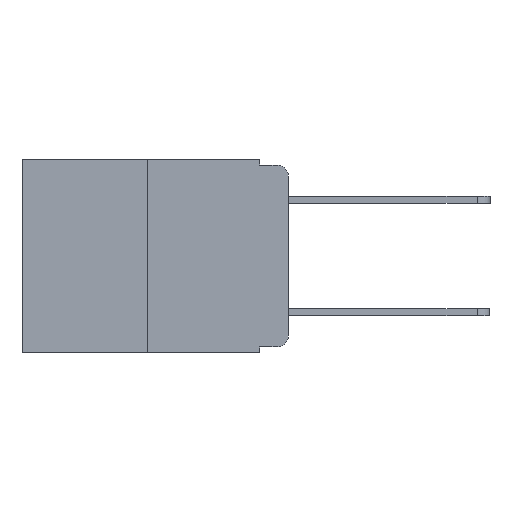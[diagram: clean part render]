
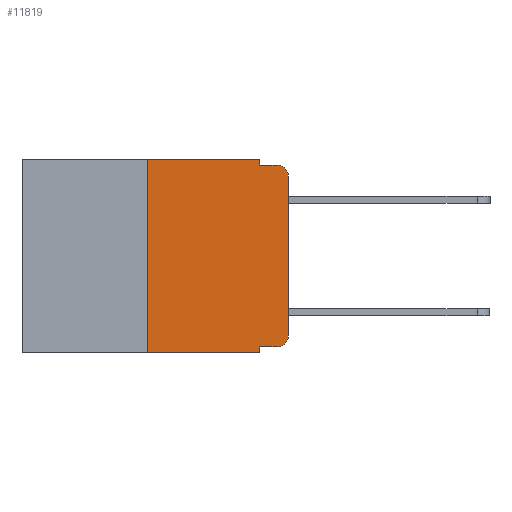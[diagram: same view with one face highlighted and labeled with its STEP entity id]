
A CAD part, left-side view. The second image highlights one B-rep face of the part: STEP entity #11819.
In plain terms, the highlighted planar face has unit normal (-1, 0, 0).
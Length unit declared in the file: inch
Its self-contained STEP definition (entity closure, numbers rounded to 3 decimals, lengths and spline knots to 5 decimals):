
#309 = LINE ( 'NONE', #13019, #859 ) ;
#859 = VECTOR ( 'NONE', #2424, 39.37008 ) ;
#1087 = CARTESIAN_POINT ( 'NONE',  ( 0., 0.051, 0. ) ) ;
#1122 = CARTESIAN_POINT ( 'NONE',  ( 0., 0.25, 0. ) ) ;
#1481 = VERTEX_POINT ( 'NONE', #22539 ) ;
#2292 = EDGE_CURVE ( 'NONE', #5380, #10473, #18486, .T. ) ;
#2424 = DIRECTION ( 'NONE',  ( 0., 0., -1. ) ) ;
#2460 = EDGE_CURVE ( 'NONE', #3141, #19604, #10316, .T. ) ;
#2606 = DIRECTION ( 'NONE',  ( -1., 0., 0. ) ) ;
#2671 = PLANE ( 'NONE',  #14979 ) ;
#3141 = VERTEX_POINT ( 'NONE', #15131 ) ;
#3881 = DIRECTION ( 'NONE',  ( 0., -1., 0. ) ) ;
#4100 = VECTOR ( 'NONE', #21245, 39.37008 ) ;
#4241 = VECTOR ( 'NONE', #3881, 39.37008 ) ;
#5121 = EDGE_CURVE ( 'NONE', #10053, #3141, #11921, .T. ) ;
#5380 = VERTEX_POINT ( 'NONE', #1122 ) ;
#5784 = ORIENTED_EDGE ( 'NONE', *, *, #21254, .F. ) ;
#5938 = EDGE_CURVE ( 'NONE', #20121, #10355, #14071, .T. ) ;
#5979 = EDGE_CURVE ( 'NONE', #11647, #5380, #17078, .T. ) ;
#6244 = DIRECTION ( 'NONE',  ( 0., 0., -1. ) ) ;
#6880 = AXIS2_PLACEMENT_3D ( 'NONE', #7999, #20255, #9759 ) ;
#7243 = CARTESIAN_POINT ( 'NONE',  ( 0., 0.02, -0.01 ) ) ;
#7429 = VECTOR ( 'NONE', #16492, 39.37008 ) ;
#7999 = CARTESIAN_POINT ( 'NONE',  ( 0., 0.02, -0.03 ) ) ;
#9759 = DIRECTION ( 'NONE',  ( 0., 0., -1. ) ) ;
#9850 = VECTOR ( 'NONE', #10065, 39.37008 ) ;
#10053 = VERTEX_POINT ( 'NONE', #13479 ) ;
#10065 = DIRECTION ( 'NONE',  ( 0., 0., -1. ) ) ;
#10316 = CIRCLE ( 'NONE', #12515, 0.02 ) ;
#10355 = VERTEX_POINT ( 'NONE', #7243 ) ;
#10473 = VERTEX_POINT ( 'NONE', #14517 ) ;
#10588 = ORIENTED_EDGE ( 'NONE', *, *, #5979, .F. ) ;
#10828 = DIRECTION ( 'NONE',  ( 0., -1., 0. ) ) ;
#11017 = EDGE_CURVE ( 'NONE', #19668, #10355, #16945, .T. ) ;
#11040 = DIRECTION ( 'NONE',  ( 0., -1., 0. ) ) ;
#11618 = CARTESIAN_POINT ( 'NONE',  ( 0., 0.25, 0. ) ) ;
#11647 = VERTEX_POINT ( 'NONE', #18071 ) ;
#11819 = ADVANCED_FACE ( 'NONE', ( #13900 ), #2671, .F. ) ;
#11921 = LINE ( 'NONE', #21492, #16004 ) ;
#12041 = ORIENTED_EDGE ( 'NONE', *, *, #5121, .T. ) ;
#12515 = AXIS2_PLACEMENT_3D ( 'NONE', #13199, #2606, #14924 ) ;
#12698 = EDGE_CURVE ( 'NONE', #10473, #19668, #309, .T. ) ;
#12857 = VECTOR ( 'NONE', #10828, 39.37008 ) ;
#13019 = CARTESIAN_POINT ( 'NONE',  ( 0., 0.051, 0. ) ) ;
#13199 = CARTESIAN_POINT ( 'NONE',  ( 0., 0.02, -0.313 ) ) ;
#13479 = CARTESIAN_POINT ( 'NONE',  ( 0., 0.051, -0.333 ) ) ;
#13900 = FACE_OUTER_BOUND ( 'NONE', #20158, .T. ) ;
#14071 = CIRCLE ( 'NONE', #6880, 0.02 ) ;
#14517 = CARTESIAN_POINT ( 'NONE',  ( 0., 0.051, 0. ) ) ;
#14591 = ORIENTED_EDGE ( 'NONE', *, *, #11017, .F. ) ;
#14723 = CARTESIAN_POINT ( 'NONE',  ( 0., 0.473, -0.343 ) ) ;
#14796 = ORIENTED_EDGE ( 'NONE', *, *, #2292, .F. ) ;
#14924 = DIRECTION ( 'NONE',  ( 0., 0., -1. ) ) ;
#14979 = AXIS2_PLACEMENT_3D ( 'NONE', #14995, #16764, #6244 ) ;
#14995 = CARTESIAN_POINT ( 'NONE',  ( 0., 0.473, 0. ) ) ;
#15058 = ORIENTED_EDGE ( 'NONE', *, *, #15961, .T. ) ;
#15069 = ORIENTED_EDGE ( 'NONE', *, *, #2460, .T. ) ;
#15091 = EDGE_CURVE ( 'NONE', #11647, #1481, #16753, .T. ) ;
#15131 = CARTESIAN_POINT ( 'NONE',  ( 0., 0.02, -0.333 ) ) ;
#15961 = EDGE_CURVE ( 'NONE', #19604, #20121, #18114, .T. ) ;
#16004 = VECTOR ( 'NONE', #11040, 39.37008 ) ;
#16492 = DIRECTION ( 'NONE',  ( 0., -1., 0. ) ) ;
#16577 = ORIENTED_EDGE ( 'NONE', *, *, #5938, .T. ) ;
#16670 = CARTESIAN_POINT ( 'NONE',  ( 0., 0.051, -0.01 ) ) ;
#16753 = LINE ( 'NONE', #14723, #7429 ) ;
#16764 = DIRECTION ( 'NONE',  ( 1., 0., 0. ) ) ;
#16945 = LINE ( 'NONE', #19546, #12857 ) ;
#17078 = LINE ( 'NONE', #11618, #17640 ) ;
#17640 = VECTOR ( 'NONE', #22066, 39.37008 ) ;
#17932 = CARTESIAN_POINT ( 'NONE',  ( 0., 0.473, 0. ) ) ;
#18071 = CARTESIAN_POINT ( 'NONE',  ( 0., 0.25, -0.343 ) ) ;
#18114 = LINE ( 'NONE', #19499, #4100 ) ;
#18125 = CARTESIAN_POINT ( 'NONE',  ( 0., 0., -0.313 ) ) ;
#18486 = LINE ( 'NONE', #17932, #4241 ) ;
#19157 = LINE ( 'NONE', #1087, #9850 ) ;
#19499 = CARTESIAN_POINT ( 'NONE',  ( 0., 0., 0. ) ) ;
#19546 = CARTESIAN_POINT ( 'NONE',  ( 0., 0.051, -0.01 ) ) ;
#19604 = VERTEX_POINT ( 'NONE', #18125 ) ;
#19668 = VERTEX_POINT ( 'NONE', #16670 ) ;
#19716 = CARTESIAN_POINT ( 'NONE',  ( 0., 0., -0.03 ) ) ;
#20121 = VERTEX_POINT ( 'NONE', #19716 ) ;
#20158 = EDGE_LOOP ( 'NONE', ( #15058, #16577, #14591, #22187, #14796, #10588, #21257, #5784, #12041, #15069 ) ) ;
#20255 = DIRECTION ( 'NONE',  ( -1., 0., 0. ) ) ;
#21245 = DIRECTION ( 'NONE',  ( 0., 0., 1. ) ) ;
#21254 = EDGE_CURVE ( 'NONE', #10053, #1481, #19157, .T. ) ;
#21257 = ORIENTED_EDGE ( 'NONE', *, *, #15091, .T. ) ;
#21492 = CARTESIAN_POINT ( 'NONE',  ( 0., 0.051, -0.333 ) ) ;
#22066 = DIRECTION ( 'NONE',  ( 0., 0., 1. ) ) ;
#22187 = ORIENTED_EDGE ( 'NONE', *, *, #12698, .F. ) ;
#22539 = CARTESIAN_POINT ( 'NONE',  ( 0., 0.051, -0.343 ) ) ;
